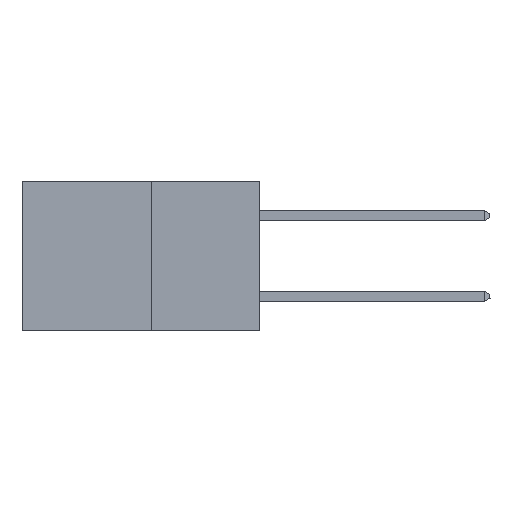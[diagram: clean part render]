
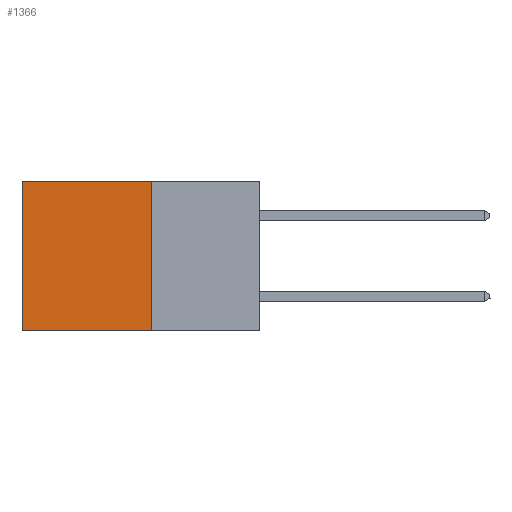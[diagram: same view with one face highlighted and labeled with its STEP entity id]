
A CAD part, left-side view. The second image highlights one B-rep face of the part: STEP entity #1366.
In plain terms, the highlighted planar face has unit normal (-1, 0, 0).
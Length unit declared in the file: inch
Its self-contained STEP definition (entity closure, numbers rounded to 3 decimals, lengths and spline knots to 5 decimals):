
#1366 = ADVANCED_FACE ( 'NONE', ( #19415 ), #15303, .F. ) ;
#2597 = CARTESIAN_POINT ( 'NONE',  ( 0.277, 0.59, 0. ) ) ;
#4832 = VECTOR ( 'NONE', #25658, 39.37008 ) ;
#5301 = DIRECTION ( 'NONE',  ( 1., 0., 0. ) ) ;
#6972 = VERTEX_POINT ( 'NONE', #32114 ) ;
#7484 = VECTOR ( 'NONE', #17257, 39.37008 ) ;
#7624 = VERTEX_POINT ( 'NONE', #15156 ) ;
#8040 = ORIENTED_EDGE ( 'NONE', *, *, #24730, .T. ) ;
#8045 = LINE ( 'NONE', #19490, #20862 ) ;
#9102 = EDGE_CURVE ( 'NONE', #6972, #7624, #12306, .T. ) ;
#9258 = EDGE_CURVE ( 'NONE', #12922, #6972, #27845, .T. ) ;
#12306 = LINE ( 'NONE', #29616, #31790 ) ;
#12922 = VERTEX_POINT ( 'NONE', #28426 ) ;
#14353 = EDGE_CURVE ( 'NONE', #27963, #7624, #8045, .T. ) ;
#15156 = CARTESIAN_POINT ( 'NONE',  ( 0.277, 0.59, -0.37 ) ) ;
#15303 = PLANE ( 'NONE',  #16912 ) ;
#16912 = AXIS2_PLACEMENT_3D ( 'NONE', #27362, #5301, #27327 ) ;
#17002 = CARTESIAN_POINT ( 'NONE',  ( 0.277, 0.27, -0.37 ) ) ;
#17231 = ORIENTED_EDGE ( 'NONE', *, *, #9258, .F. ) ;
#17257 = DIRECTION ( 'NONE',  ( 0., 0., -1. ) ) ;
#18549 = LINE ( 'NONE', #23099, #4832 ) ;
#19415 = FACE_OUTER_BOUND ( 'NONE', #27581, .T. ) ;
#19490 = CARTESIAN_POINT ( 'NONE',  ( 0.277, 0.59, -0.37 ) ) ;
#20862 = VECTOR ( 'NONE', #24543, 39.37008 ) ;
#23099 = CARTESIAN_POINT ( 'NONE',  ( 0.277, 0.27, 0. ) ) ;
#23572 = ORIENTED_EDGE ( 'NONE', *, *, #14353, .T. ) ;
#24543 = DIRECTION ( 'NONE',  ( 0., 0., -1. ) ) ;
#24730 = EDGE_CURVE ( 'NONE', #12922, #27963, #18549, .T. ) ;
#25658 = DIRECTION ( 'NONE',  ( 0., 1., 0. ) ) ;
#27088 = ORIENTED_EDGE ( 'NONE', *, *, #9102, .F. ) ;
#27327 = DIRECTION ( 'NONE',  ( 0., 0., -1. ) ) ;
#27362 = CARTESIAN_POINT ( 'NONE',  ( 0.277, 0.27, -0.37 ) ) ;
#27581 = EDGE_LOOP ( 'NONE', ( #23572, #27088, #17231, #8040 ) ) ;
#27845 = LINE ( 'NONE', #17002, #7484 ) ;
#27963 = VERTEX_POINT ( 'NONE', #2597 ) ;
#28369 = DIRECTION ( 'NONE',  ( 0., 1., 0. ) ) ;
#28426 = CARTESIAN_POINT ( 'NONE',  ( 0.277, 0.27, 0. ) ) ;
#29616 = CARTESIAN_POINT ( 'NONE',  ( 0.277, 0.27, -0.37 ) ) ;
#31790 = VECTOR ( 'NONE', #28369, 39.37008 ) ;
#32114 = CARTESIAN_POINT ( 'NONE',  ( 0.277, 0.27, -0.37 ) ) ;
